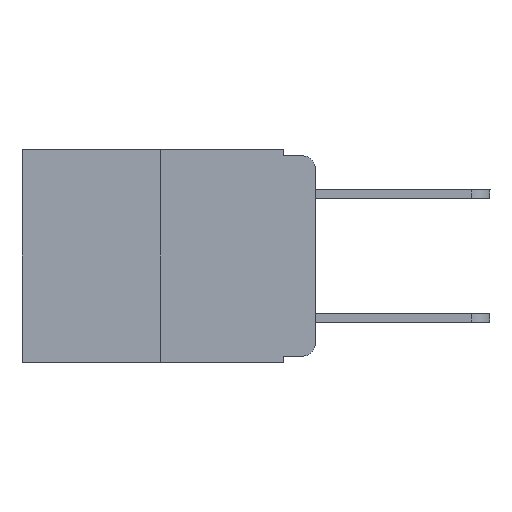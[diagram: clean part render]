
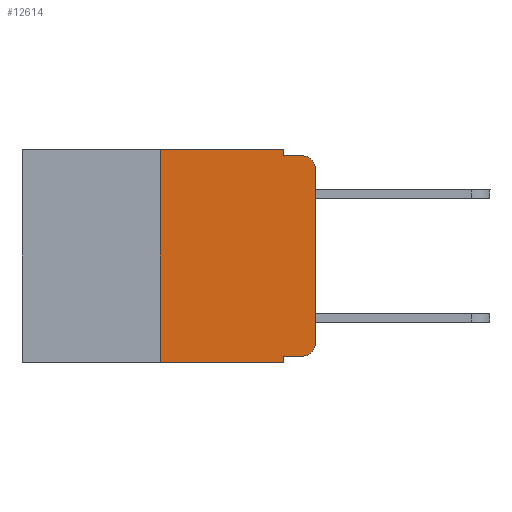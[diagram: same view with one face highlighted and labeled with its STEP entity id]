
A CAD part, left-side view. The second image highlights one B-rep face of the part: STEP entity #12614.
In plain terms, the highlighted planar face has unit normal (-1, 0, 0).
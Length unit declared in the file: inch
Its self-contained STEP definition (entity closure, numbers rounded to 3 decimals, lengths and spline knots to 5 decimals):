
#96 = CARTESIAN_POINT ( 'NONE',  ( 0., 0.473, 0. ) ) ;
#277 = DIRECTION ( 'NONE',  ( 0., -1., 0. ) ) ;
#505 = CARTESIAN_POINT ( 'NONE',  ( 0., 0.051, 0. ) ) ;
#511 = AXIS2_PLACEMENT_3D ( 'NONE', #13190, #15865, #916 ) ;
#636 = VECTOR ( 'NONE', #2942, 39.37008 ) ;
#916 = DIRECTION ( 'NONE',  ( 0., 0., -1. ) ) ;
#939 = EDGE_CURVE ( 'NONE', #5966, #8899, #3839, .T. ) ;
#1320 = EDGE_LOOP ( 'NONE', ( #4665, #3592, #6548, #8395, #5261, #6794, #2517, #7519, #4017, #11990 ) ) ;
#1508 = DIRECTION ( 'NONE',  ( 0., -1., 0. ) ) ;
#2010 = CARTESIAN_POINT ( 'NONE',  ( 0., 0.051, -0.01 ) ) ;
#2336 = LINE ( 'NONE', #6183, #14840 ) ;
#2517 = ORIENTED_EDGE ( 'NONE', *, *, #11447, .T. ) ;
#2523 = EDGE_CURVE ( 'NONE', #7926, #14460, #4371, .T. ) ;
#2551 = CARTESIAN_POINT ( 'NONE',  ( 0., 0.051, 0. ) ) ;
#2736 = EDGE_CURVE ( 'NONE', #14197, #5966, #13505, .T. ) ;
#2942 = DIRECTION ( 'NONE',  ( 0., 0., -1. ) ) ;
#3000 = VERTEX_POINT ( 'NONE', #2010 ) ;
#3592 = ORIENTED_EDGE ( 'NONE', *, *, #5500, .T. ) ;
#3622 = VECTOR ( 'NONE', #277, 39.37008 ) ;
#3839 = CIRCLE ( 'NONE', #10737, 0.02 ) ;
#3856 = CARTESIAN_POINT ( 'NONE',  ( 0., 0., -0.03 ) ) ;
#4006 = LINE ( 'NONE', #8954, #4355 ) ;
#4017 = ORIENTED_EDGE ( 'NONE', *, *, #2736, .T. ) ;
#4031 = LINE ( 'NONE', #12625, #14132 ) ;
#4044 = EDGE_CURVE ( 'NONE', #14197, #15692, #12770, .T. ) ;
#4286 = EDGE_CURVE ( 'NONE', #14460, #13737, #10009, .T. ) ;
#4355 = VECTOR ( 'NONE', #1508, 39.37008 ) ;
#4371 = LINE ( 'NONE', #12794, #10485 ) ;
#4536 = CARTESIAN_POINT ( 'NONE',  ( 0., 0.25, 0. ) ) ;
#4665 = ORIENTED_EDGE ( 'NONE', *, *, #7386, .T. ) ;
#4694 = CARTESIAN_POINT ( 'NONE',  ( 0., 0.02, -0.03 ) ) ;
#5247 = EDGE_CURVE ( 'NONE', #13737, #3000, #12719, .T. ) ;
#5261 = ORIENTED_EDGE ( 'NONE', *, *, #4286, .F. ) ;
#5500 = EDGE_CURVE ( 'NONE', #14977, #7057, #9104, .T. ) ;
#5966 = VERTEX_POINT ( 'NONE', #12345 ) ;
#6183 = CARTESIAN_POINT ( 'NONE',  ( 0., 0., 0. ) ) ;
#6548 = ORIENTED_EDGE ( 'NONE', *, *, #12499, .F. ) ;
#6794 = ORIENTED_EDGE ( 'NONE', *, *, #2523, .F. ) ;
#6865 = CARTESIAN_POINT ( 'NONE',  ( 0., 0., -0.313 ) ) ;
#7057 = VERTEX_POINT ( 'NONE', #11401 ) ;
#7261 = DIRECTION ( 'NONE',  ( -1., 0., 0. ) ) ;
#7386 = EDGE_CURVE ( 'NONE', #8899, #14977, #2336, .T. ) ;
#7504 = DIRECTION ( 'NONE',  ( 0., 0., -1. ) ) ;
#7519 = ORIENTED_EDGE ( 'NONE', *, *, #4044, .F. ) ;
#7870 = DIRECTION ( 'NONE',  ( 0., -1., 0. ) ) ;
#7926 = VERTEX_POINT ( 'NONE', #11180 ) ;
#8083 = AXIS2_PLACEMENT_3D ( 'NONE', #4694, #14237, #9488 ) ;
#8145 = CARTESIAN_POINT ( 'NONE',  ( 0., 0.02, -0.313 ) ) ;
#8395 = ORIENTED_EDGE ( 'NONE', *, *, #5247, .F. ) ;
#8479 = CARTESIAN_POINT ( 'NONE',  ( 0., 0.051, -0.333 ) ) ;
#8767 = CARTESIAN_POINT ( 'NONE',  ( 0., 0.051, -0.333 ) ) ;
#8899 = VERTEX_POINT ( 'NONE', #6865 ) ;
#8954 = CARTESIAN_POINT ( 'NONE',  ( 0., 0.051, -0.01 ) ) ;
#9104 = CIRCLE ( 'NONE', #8083, 0.02 ) ;
#9258 = DIRECTION ( 'NONE',  ( 0., 0., 1. ) ) ;
#9341 = CARTESIAN_POINT ( 'NONE',  ( 0., 0.051, -0.343 ) ) ;
#9488 = DIRECTION ( 'NONE',  ( 0., 0., -1. ) ) ;
#9855 = DIRECTION ( 'NONE',  ( 0., 0., 1. ) ) ;
#10009 = LINE ( 'NONE', #96, #15552 ) ;
#10115 = VECTOR ( 'NONE', #14152, 39.37008 ) ;
#10485 = VECTOR ( 'NONE', #9258, 39.37008 ) ;
#10605 = PLANE ( 'NONE',  #511 ) ;
#10737 = AXIS2_PLACEMENT_3D ( 'NONE', #8145, #7261, #7504 ) ;
#10971 = DIRECTION ( 'NONE',  ( 0., -1., 0. ) ) ;
#11180 = CARTESIAN_POINT ( 'NONE',  ( 0., 0.25, -0.343 ) ) ;
#11401 = CARTESIAN_POINT ( 'NONE',  ( 0., 0.02, -0.01 ) ) ;
#11447 = EDGE_CURVE ( 'NONE', #7926, #15692, #4031, .T. ) ;
#11990 = ORIENTED_EDGE ( 'NONE', *, *, #939, .T. ) ;
#12345 = CARTESIAN_POINT ( 'NONE',  ( 0., 0.02, -0.333 ) ) ;
#12499 = EDGE_CURVE ( 'NONE', #3000, #7057, #4006, .T. ) ;
#12614 = ADVANCED_FACE ( 'NONE', ( #13356 ), #10605, .F. ) ;
#12625 = CARTESIAN_POINT ( 'NONE',  ( 0., 0.473, -0.343 ) ) ;
#12719 = LINE ( 'NONE', #12792, #636 ) ;
#12770 = LINE ( 'NONE', #505, #10115 ) ;
#12792 = CARTESIAN_POINT ( 'NONE',  ( 0., 0.051, 0. ) ) ;
#12794 = CARTESIAN_POINT ( 'NONE',  ( 0., 0.25, 0. ) ) ;
#13190 = CARTESIAN_POINT ( 'NONE',  ( 0., 0.473, 0. ) ) ;
#13356 = FACE_OUTER_BOUND ( 'NONE', #1320, .T. ) ;
#13505 = LINE ( 'NONE', #8767, #3622 ) ;
#13737 = VERTEX_POINT ( 'NONE', #2551 ) ;
#14132 = VECTOR ( 'NONE', #7870, 39.37008 ) ;
#14152 = DIRECTION ( 'NONE',  ( 0., 0., -1. ) ) ;
#14197 = VERTEX_POINT ( 'NONE', #8479 ) ;
#14237 = DIRECTION ( 'NONE',  ( -1., 0., 0. ) ) ;
#14460 = VERTEX_POINT ( 'NONE', #4536 ) ;
#14840 = VECTOR ( 'NONE', #9855, 39.37008 ) ;
#14977 = VERTEX_POINT ( 'NONE', #3856 ) ;
#15552 = VECTOR ( 'NONE', #10971, 39.37008 ) ;
#15692 = VERTEX_POINT ( 'NONE', #9341 ) ;
#15865 = DIRECTION ( 'NONE',  ( 1., 0., 0. ) ) ;
